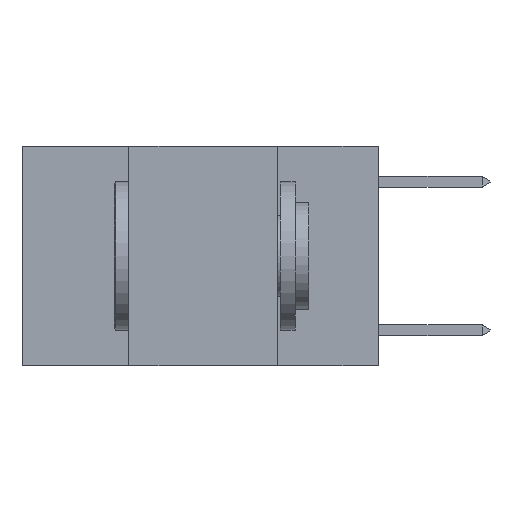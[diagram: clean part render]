
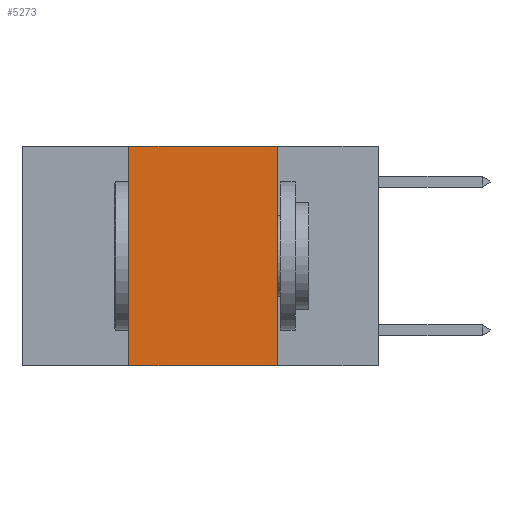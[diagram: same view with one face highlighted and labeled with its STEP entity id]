
A CAD part, left-side view. The second image highlights one B-rep face of the part: STEP entity #5273.
In plain terms, the highlighted planar face has unit normal (-1, 0, 0).
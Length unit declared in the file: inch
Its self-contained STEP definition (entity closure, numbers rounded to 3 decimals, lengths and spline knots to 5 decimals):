
#1693 = CARTESIAN_POINT ( 'NONE',  ( 0., 0.42, 0. ) ) ;
#2375 = VERTEX_POINT ( 'NONE', #19150 ) ;
#2760 = DIRECTION ( 'NONE',  ( 0., 0., -1. ) ) ;
#3064 = CARTESIAN_POINT ( 'NONE',  ( 0., 0.17, -0.37 ) ) ;
#3353 = LINE ( 'NONE', #22399, #24297 ) ;
#4193 = VERTEX_POINT ( 'NONE', #17513 ) ;
#4947 = DIRECTION ( 'NONE',  ( 0., -1., 0. ) ) ;
#5273 = ADVANCED_FACE ( 'NONE', ( #22889 ), #7712, .F. ) ;
#6087 = CARTESIAN_POINT ( 'NONE',  ( 0., 0.6, 0. ) ) ;
#6284 = VECTOR ( 'NONE', #2760, 39.37008 ) ;
#6559 = EDGE_CURVE ( 'NONE', #24300, #2375, #15261, .T. ) ;
#7052 = EDGE_LOOP ( 'NONE', ( #10658, #23604, #16828, #10821 ) ) ;
#7712 = PLANE ( 'NONE',  #15240 ) ;
#8651 = VECTOR ( 'NONE', #11296, 39.37008 ) ;
#8809 = CARTESIAN_POINT ( 'NONE',  ( 0., 0.6, 0. ) ) ;
#10187 = VERTEX_POINT ( 'NONE', #3064 ) ;
#10449 = EDGE_CURVE ( 'NONE', #4193, #10187, #22165, .T. ) ;
#10658 = ORIENTED_EDGE ( 'NONE', *, *, #10449, .F. ) ;
#10821 = ORIENTED_EDGE ( 'NONE', *, *, #23984, .T. ) ;
#10959 = DIRECTION ( 'NONE',  ( 0., -1., 0. ) ) ;
#11296 = DIRECTION ( 'NONE',  ( 0., 0., 1. ) ) ;
#11302 = VECTOR ( 'NONE', #4947, 39.37008 ) ;
#11574 = DIRECTION ( 'NONE',  ( 0., 0., -1. ) ) ;
#11699 = DIRECTION ( 'NONE',  ( 1., 0., 0. ) ) ;
#12482 = CARTESIAN_POINT ( 'NONE',  ( 0., 0.17, 0. ) ) ;
#15240 = AXIS2_PLACEMENT_3D ( 'NONE', #6087, #11699, #11574 ) ;
#15261 = LINE ( 'NONE', #1693, #8651 ) ;
#16133 = LINE ( 'NONE', #8809, #11302 ) ;
#16828 = ORIENTED_EDGE ( 'NONE', *, *, #6559, .F. ) ;
#17513 = CARTESIAN_POINT ( 'NONE',  ( 0., 0.17, 0. ) ) ;
#19150 = CARTESIAN_POINT ( 'NONE',  ( 0., 0.42, 0. ) ) ;
#19272 = EDGE_CURVE ( 'NONE', #2375, #4193, #16133, .T. ) ;
#22165 = LINE ( 'NONE', #12482, #6284 ) ;
#22399 = CARTESIAN_POINT ( 'NONE',  ( 0., 0.6, -0.37 ) ) ;
#22889 = FACE_OUTER_BOUND ( 'NONE', #7052, .T. ) ;
#23125 = CARTESIAN_POINT ( 'NONE',  ( 0., 0.42, -0.37 ) ) ;
#23604 = ORIENTED_EDGE ( 'NONE', *, *, #19272, .F. ) ;
#23984 = EDGE_CURVE ( 'NONE', #24300, #10187, #3353, .T. ) ;
#24297 = VECTOR ( 'NONE', #10959, 39.37008 ) ;
#24300 = VERTEX_POINT ( 'NONE', #23125 ) ;
